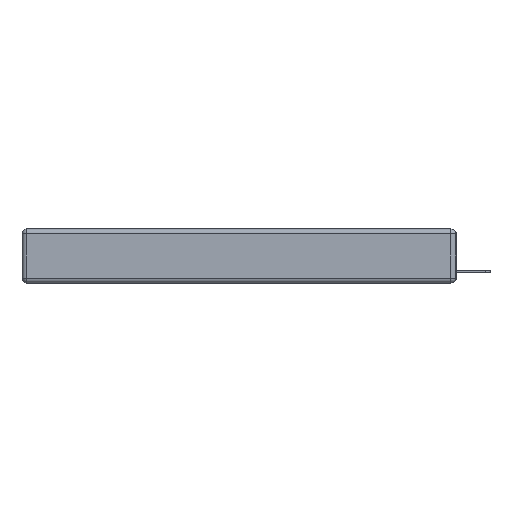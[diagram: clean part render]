
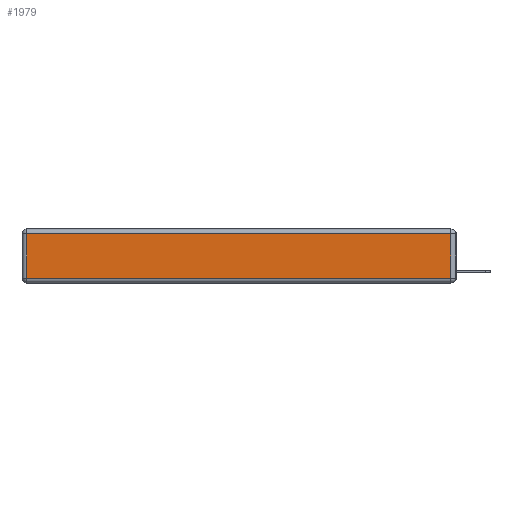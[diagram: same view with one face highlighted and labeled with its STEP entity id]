
A CAD part, left-side view. The second image highlights one B-rep face of the part: STEP entity #1979.
In plain terms, the highlighted planar face has unit normal (-1, 0, 0).
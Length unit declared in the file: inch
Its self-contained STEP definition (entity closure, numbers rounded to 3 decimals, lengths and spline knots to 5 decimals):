
#24 = DIRECTION ( 'NONE',  ( -1., 0., 0. ) ) ;
#25 = EDGE_LOOP ( 'NONE', ( #7469, #10153, #7433, #2358 ) ) ;
#1979 = ADVANCED_FACE ( 'NONE', ( #10109 ), #5715, .T. ) ;
#2179 = EDGE_CURVE ( 'NONE', #13619, #9114, #13993, .T. ) ;
#2356 = CARTESIAN_POINT ( 'NONE',  ( 0., 0.03, -0.343 ) ) ;
#2358 = ORIENTED_EDGE ( 'NONE', *, *, #11988, .T. ) ;
#2473 = VERTEX_POINT ( 'NONE', #5606 ) ;
#2936 = CARTESIAN_POINT ( 'NONE',  ( 0., 2.75, -0.03 ) ) ;
#3335 = LINE ( 'NONE', #2356, #12788 ) ;
#4018 = DIRECTION ( 'NONE',  ( 0., 1., 0. ) ) ;
#4271 = EDGE_CURVE ( 'NONE', #9114, #4979, #3335, .T. ) ;
#4354 = VECTOR ( 'NONE', #4018, 39.37008 ) ;
#4979 = VERTEX_POINT ( 'NONE', #14352 ) ;
#5606 = CARTESIAN_POINT ( 'NONE',  ( 0., 2.72, -0.03 ) ) ;
#5715 = PLANE ( 'NONE',  #13854 ) ;
#6958 = VECTOR ( 'NONE', #12008, 39.37008 ) ;
#7381 = EDGE_CURVE ( 'NONE', #4979, #2473, #10517, .T. ) ;
#7433 = ORIENTED_EDGE ( 'NONE', *, *, #7381, .T. ) ;
#7469 = ORIENTED_EDGE ( 'NONE', *, *, #2179, .T. ) ;
#7639 = CARTESIAN_POINT ( 'NONE',  ( 0., 0.03, -0.313 ) ) ;
#8354 = CARTESIAN_POINT ( 'NONE',  ( 0., 2.72, -0.313 ) ) ;
#9114 = VERTEX_POINT ( 'NONE', #7639 ) ;
#10020 = CARTESIAN_POINT ( 'NONE',  ( 0., 2.72, -0.343 ) ) ;
#10109 = FACE_OUTER_BOUND ( 'NONE', #25, .T. ) ;
#10153 = ORIENTED_EDGE ( 'NONE', *, *, #4271, .T. ) ;
#10517 = LINE ( 'NONE', #2936, #4354 ) ;
#10824 = CARTESIAN_POINT ( 'NONE',  ( 0., 0., -0.313 ) ) ;
#11650 = DIRECTION ( 'NONE',  ( 0., 0., 1. ) ) ;
#11876 = VECTOR ( 'NONE', #14706, 39.37008 ) ;
#11885 = DIRECTION ( 'NONE',  ( 0., 0., 1. ) ) ;
#11988 = EDGE_CURVE ( 'NONE', #2473, #13619, #12229, .T. ) ;
#12008 = DIRECTION ( 'NONE',  ( 0., -1., 0. ) ) ;
#12229 = LINE ( 'NONE', #10020, #11876 ) ;
#12788 = VECTOR ( 'NONE', #11885, 39.37008 ) ;
#12831 = CARTESIAN_POINT ( 'NONE',  ( 0., 0., -0.343 ) ) ;
#13619 = VERTEX_POINT ( 'NONE', #8354 ) ;
#13854 = AXIS2_PLACEMENT_3D ( 'NONE', #12831, #24, #11650 ) ;
#13993 = LINE ( 'NONE', #10824, #6958 ) ;
#14352 = CARTESIAN_POINT ( 'NONE',  ( 0., 0.03, -0.03 ) ) ;
#14706 = DIRECTION ( 'NONE',  ( 0., 0., -1. ) ) ;
